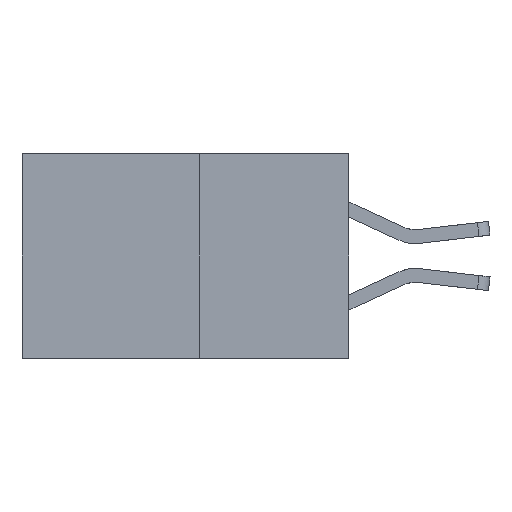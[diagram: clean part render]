
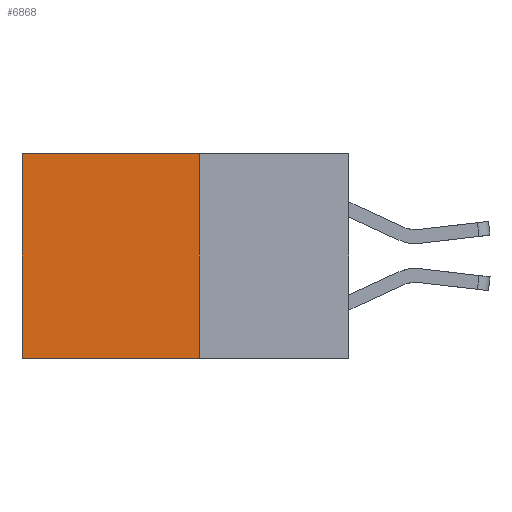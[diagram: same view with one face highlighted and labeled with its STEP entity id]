
A CAD part, left-side view. The second image highlights one B-rep face of the part: STEP entity #6868.
In plain terms, the highlighted planar face has unit normal (-1, 0, 0).
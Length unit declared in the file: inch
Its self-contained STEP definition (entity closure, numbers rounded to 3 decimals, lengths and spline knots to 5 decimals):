
#152 = EDGE_CURVE ( 'NONE', #7971, #6144, #8561, .T. ) ;
#160 = DIRECTION ( 'NONE',  ( 0., 0., -1. ) ) ;
#635 = EDGE_CURVE ( 'NONE', #7971, #4663, #1110, .T. ) ;
#777 = CARTESIAN_POINT ( 'NONE',  ( 0.277, 0.27, -0.37 ) ) ;
#938 = EDGE_CURVE ( 'NONE', #4663, #4583, #8540, .T. ) ;
#967 = CARTESIAN_POINT ( 'NONE',  ( 0.277, 0.59, 0. ) ) ;
#1110 = LINE ( 'NONE', #1207, #4575 ) ;
#1207 = CARTESIAN_POINT ( 'NONE',  ( 0.277, 0.27, 0. ) ) ;
#1568 = CARTESIAN_POINT ( 'NONE',  ( 0.277, 0.59, -0.37 ) ) ;
#1638 = DIRECTION ( 'NONE',  ( 0., 0., -1. ) ) ;
#2469 = VECTOR ( 'NONE', #4730, 39.37008 ) ;
#2697 = ORIENTED_EDGE ( 'NONE', *, *, #152, .F. ) ;
#3064 = VECTOR ( 'NONE', #160, 39.37008 ) ;
#4338 = PLANE ( 'NONE',  #5959 ) ;
#4459 = CARTESIAN_POINT ( 'NONE',  ( 0.277, 0.27, 0. ) ) ;
#4536 = DIRECTION ( 'NONE',  ( 0., 0., -1. ) ) ;
#4575 = VECTOR ( 'NONE', #5379, 39.37008 ) ;
#4583 = VERTEX_POINT ( 'NONE', #1568 ) ;
#4663 = VERTEX_POINT ( 'NONE', #967 ) ;
#4689 = ORIENTED_EDGE ( 'NONE', *, *, #635, .T. ) ;
#4730 = DIRECTION ( 'NONE',  ( 0., 1., 0. ) ) ;
#4985 = FACE_OUTER_BOUND ( 'NONE', #7863, .T. ) ;
#5075 = CARTESIAN_POINT ( 'NONE',  ( 0.277, 0.59, -0.37 ) ) ;
#5379 = DIRECTION ( 'NONE',  ( 0., 1., 0. ) ) ;
#5445 = EDGE_CURVE ( 'NONE', #6144, #4583, #8230, .T. ) ;
#5959 = AXIS2_PLACEMENT_3D ( 'NONE', #7391, #7541, #4536 ) ;
#6144 = VERTEX_POINT ( 'NONE', #8165 ) ;
#6476 = VECTOR ( 'NONE', #1638, 39.37008 ) ;
#6868 = ADVANCED_FACE ( 'NONE', ( #4985 ), #4338, .F. ) ;
#7187 = CARTESIAN_POINT ( 'NONE',  ( 0.277, 0.27, -0.37 ) ) ;
#7299 = ORIENTED_EDGE ( 'NONE', *, *, #5445, .F. ) ;
#7391 = CARTESIAN_POINT ( 'NONE',  ( 0.277, 0.27, -0.37 ) ) ;
#7541 = DIRECTION ( 'NONE',  ( 1., 0., 0. ) ) ;
#7863 = EDGE_LOOP ( 'NONE', ( #8120, #7299, #2697, #4689 ) ) ;
#7971 = VERTEX_POINT ( 'NONE', #4459 ) ;
#8120 = ORIENTED_EDGE ( 'NONE', *, *, #938, .T. ) ;
#8165 = CARTESIAN_POINT ( 'NONE',  ( 0.277, 0.27, -0.37 ) ) ;
#8230 = LINE ( 'NONE', #7187, #2469 ) ;
#8540 = LINE ( 'NONE', #5075, #6476 ) ;
#8561 = LINE ( 'NONE', #777, #3064 ) ;
